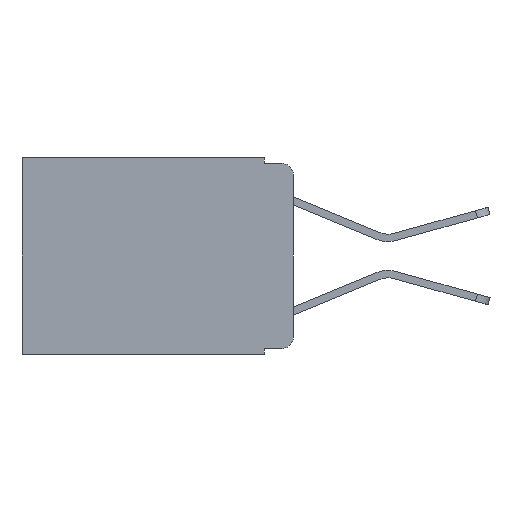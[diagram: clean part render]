
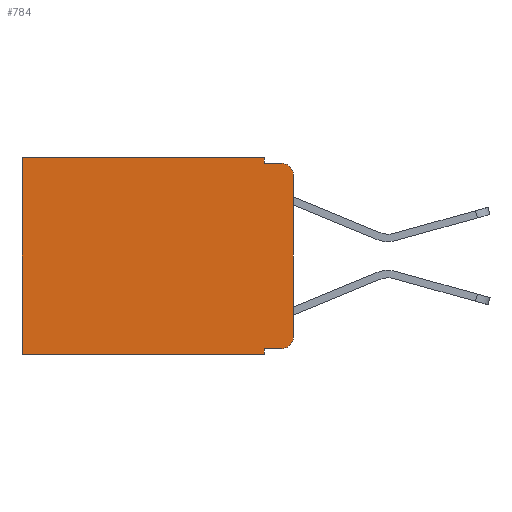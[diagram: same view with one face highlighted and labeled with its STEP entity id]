
A CAD part, left-side view. The second image highlights one B-rep face of the part: STEP entity #784.
In plain terms, the highlighted planar face has unit normal (-1, 0, 0).
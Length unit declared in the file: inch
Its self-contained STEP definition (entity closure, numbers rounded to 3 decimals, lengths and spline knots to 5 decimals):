
#32 = CARTESIAN_POINT ( 'NONE',  ( 0.298, 0.051, -0.01 ) ) ;
#343 = EDGE_CURVE ( 'NONE', #6243, #12002, #4994, .T. ) ;
#489 = DIRECTION ( 'NONE',  ( 0., 0., -1. ) ) ;
#628 = VERTEX_POINT ( 'NONE', #8224 ) ;
#632 = LINE ( 'NONE', #1192, #11811 ) ;
#645 = EDGE_CURVE ( 'NONE', #628, #6243, #1589, .T. ) ;
#683 = EDGE_CURVE ( 'NONE', #11206, #8999, #5737, .T. ) ;
#784 = ADVANCED_FACE ( 'NONE', ( #1285 ), #12437, .F. ) ;
#833 = VECTOR ( 'NONE', #489, 39.37008 ) ;
#1041 = CARTESIAN_POINT ( 'NONE',  ( 0.298, 0., -0.343 ) ) ;
#1192 = CARTESIAN_POINT ( 'NONE',  ( 0.298, 0.051, 0. ) ) ;
#1233 = ORIENTED_EDGE ( 'NONE', *, *, #645, .F. ) ;
#1285 = FACE_OUTER_BOUND ( 'NONE', #5833, .T. ) ;
#1324 = ORIENTED_EDGE ( 'NONE', *, *, #8830, .F. ) ;
#1428 = AXIS2_PLACEMENT_3D ( 'NONE', #3664, #8623, #2729 ) ;
#1589 = LINE ( 'NONE', #6312, #8339 ) ;
#2049 = EDGE_CURVE ( 'NONE', #4688, #6582, #3882, .T. ) ;
#2240 = CARTESIAN_POINT ( 'NONE',  ( 0.298, 0.02, -0.01 ) ) ;
#2283 = EDGE_CURVE ( 'NONE', #7455, #8999, #6498, .T. ) ;
#2562 = DIRECTION ( 'NONE',  ( 1., 0., 0. ) ) ;
#2729 = DIRECTION ( 'NONE',  ( 0., 0., -1. ) ) ;
#2835 = VECTOR ( 'NONE', #10228, 39.37008 ) ;
#2991 = VECTOR ( 'NONE', #6514, 39.37008 ) ;
#2993 = VERTEX_POINT ( 'NONE', #2240 ) ;
#3021 = ORIENTED_EDGE ( 'NONE', *, *, #2283, .T. ) ;
#3037 = CARTESIAN_POINT ( 'NONE',  ( 0.298, 0., 0. ) ) ;
#3293 = CARTESIAN_POINT ( 'NONE',  ( 0.298, 0.02, -0.333 ) ) ;
#3363 = ORIENTED_EDGE ( 'NONE', *, *, #683, .F. ) ;
#3394 = VERTEX_POINT ( 'NONE', #32 ) ;
#3555 = ORIENTED_EDGE ( 'NONE', *, *, #11405, .F. ) ;
#3664 = CARTESIAN_POINT ( 'NONE',  ( 0.298, 0.02, -0.03 ) ) ;
#3725 = DIRECTION ( 'NONE',  ( -1., 0., 0. ) ) ;
#3882 = LINE ( 'NONE', #3037, #6784 ) ;
#4079 = DIRECTION ( 'NONE',  ( 0., 0., -1. ) ) ;
#4355 = VECTOR ( 'NONE', #5282, 39.37008 ) ;
#4516 = LINE ( 'NONE', #12189, #2835 ) ;
#4576 = ORIENTED_EDGE ( 'NONE', *, *, #2049, .T. ) ;
#4688 = VERTEX_POINT ( 'NONE', #12101 ) ;
#4957 = EDGE_CURVE ( 'NONE', #11206, #2993, #12677, .T. ) ;
#4994 = LINE ( 'NONE', #1041, #11700 ) ;
#5101 = DIRECTION ( 'NONE',  ( 0., 1., 0. ) ) ;
#5282 = DIRECTION ( 'NONE',  ( 0., 0., -1. ) ) ;
#5311 = LINE ( 'NONE', #8498, #2991 ) ;
#5737 = LINE ( 'NONE', #11272, #833 ) ;
#5833 = EDGE_LOOP ( 'NONE', ( #3363, #8557, #1324, #3555, #4576, #11183, #6077, #1233, #6177, #3021 ) ) ;
#5930 = LINE ( 'NONE', #11433, #4355 ) ;
#6077 = ORIENTED_EDGE ( 'NONE', *, *, #343, .F. ) ;
#6177 = ORIENTED_EDGE ( 'NONE', *, *, #7379, .T. ) ;
#6243 = VERTEX_POINT ( 'NONE', #6380 ) ;
#6312 = CARTESIAN_POINT ( 'NONE',  ( 0.298, 0.051, 0. ) ) ;
#6380 = CARTESIAN_POINT ( 'NONE',  ( 0.298, 0.051, -0.343 ) ) ;
#6498 = CIRCLE ( 'NONE', #11163, 0.02 ) ;
#6514 = DIRECTION ( 'NONE',  ( 0., -1., 0. ) ) ;
#6582 = VERTEX_POINT ( 'NONE', #10084 ) ;
#6784 = VECTOR ( 'NONE', #5101, 39.37008 ) ;
#7379 = EDGE_CURVE ( 'NONE', #628, #7455, #5311, .T. ) ;
#7455 = VERTEX_POINT ( 'NONE', #3293 ) ;
#7459 = EDGE_CURVE ( 'NONE', #6582, #12002, #5930, .T. ) ;
#7638 = CARTESIAN_POINT ( 'NONE',  ( 0.298, 0., -0.03 ) ) ;
#7791 = DIRECTION ( 'NONE',  ( 0., 1., 0. ) ) ;
#8224 = CARTESIAN_POINT ( 'NONE',  ( 0.298, 0.051, -0.333 ) ) ;
#8339 = VECTOR ( 'NONE', #10236, 39.37008 ) ;
#8498 = CARTESIAN_POINT ( 'NONE',  ( 0.298, 0.051, -0.333 ) ) ;
#8499 = CARTESIAN_POINT ( 'NONE',  ( 0.298, 0., 0. ) ) ;
#8557 = ORIENTED_EDGE ( 'NONE', *, *, #4957, .T. ) ;
#8623 = DIRECTION ( 'NONE',  ( -1., 0., 0. ) ) ;
#8789 = CARTESIAN_POINT ( 'NONE',  ( 0.298, 0., -0.313 ) ) ;
#8830 = EDGE_CURVE ( 'NONE', #3394, #2993, #4516, .T. ) ;
#8999 = VERTEX_POINT ( 'NONE', #8789 ) ;
#9603 = CARTESIAN_POINT ( 'NONE',  ( 0.298, 0.02, -0.313 ) ) ;
#10084 = CARTESIAN_POINT ( 'NONE',  ( 0.298, 0.473, 0. ) ) ;
#10228 = DIRECTION ( 'NONE',  ( 0., -1., 0. ) ) ;
#10236 = DIRECTION ( 'NONE',  ( 0., 0., -1. ) ) ;
#10456 = DIRECTION ( 'NONE',  ( 0., 0., -1. ) ) ;
#10585 = DIRECTION ( 'NONE',  ( 0., 0., -1. ) ) ;
#11163 = AXIS2_PLACEMENT_3D ( 'NONE', #9603, #3725, #10585 ) ;
#11183 = ORIENTED_EDGE ( 'NONE', *, *, #7459, .T. ) ;
#11206 = VERTEX_POINT ( 'NONE', #7638 ) ;
#11272 = CARTESIAN_POINT ( 'NONE',  ( 0.298, 0., 0. ) ) ;
#11405 = EDGE_CURVE ( 'NONE', #4688, #3394, #632, .T. ) ;
#11433 = CARTESIAN_POINT ( 'NONE',  ( 0.298, 0.473, 0. ) ) ;
#11626 = AXIS2_PLACEMENT_3D ( 'NONE', #8499, #2562, #10456 ) ;
#11700 = VECTOR ( 'NONE', #7791, 39.37008 ) ;
#11701 = CARTESIAN_POINT ( 'NONE',  ( 0.298, 0.473, -0.343 ) ) ;
#11811 = VECTOR ( 'NONE', #4079, 39.37008 ) ;
#12002 = VERTEX_POINT ( 'NONE', #11701 ) ;
#12101 = CARTESIAN_POINT ( 'NONE',  ( 0.298, 0.051, 0. ) ) ;
#12189 = CARTESIAN_POINT ( 'NONE',  ( 0.298, 0.051, -0.01 ) ) ;
#12437 = PLANE ( 'NONE',  #11626 ) ;
#12677 = CIRCLE ( 'NONE', #1428, 0.02 ) ;
